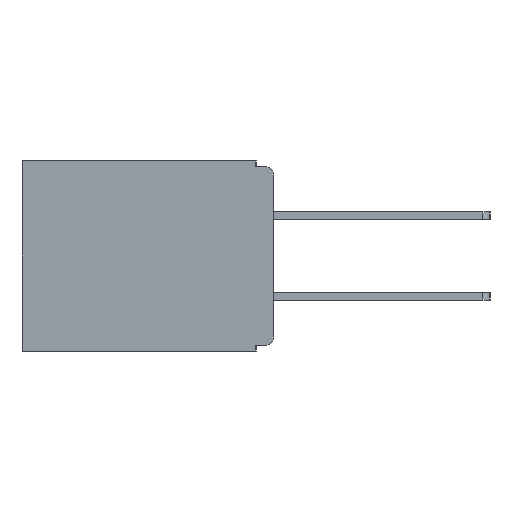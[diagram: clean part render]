
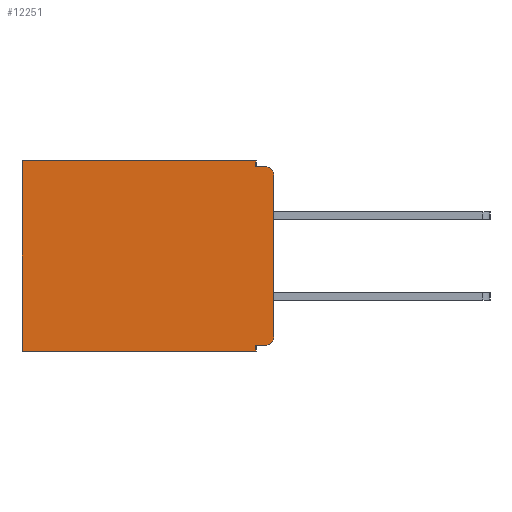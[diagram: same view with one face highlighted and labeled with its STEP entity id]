
A CAD part, left-side view. The second image highlights one B-rep face of the part: STEP entity #12251.
In plain terms, the highlighted planar face has unit normal (-1, 0, 0).
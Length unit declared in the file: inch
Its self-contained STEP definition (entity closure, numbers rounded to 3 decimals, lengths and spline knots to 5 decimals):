
#84 = AXIS2_PLACEMENT_3D ( 'NONE', #14376, #28313, #7454 ) ;
#860 = CARTESIAN_POINT ( 'NONE',  ( 0.3, 0.437, 0. ) ) ;
#1020 = DIRECTION ( 'NONE',  ( 0., 1., 0. ) ) ;
#1038 = CARTESIAN_POINT ( 'NONE',  ( 0.3, 0.015, -0.01 ) ) ;
#1476 = DIRECTION ( 'NONE',  ( 0., 0., -1. ) ) ;
#2027 = CARTESIAN_POINT ( 'NONE',  ( 0.3, 0.031, -0.32 ) ) ;
#2091 = EDGE_CURVE ( 'NONE', #27641, #7445, #16041, .T. ) ;
#2243 = CARTESIAN_POINT ( 'NONE',  ( 0.3, 0.031, -0.01 ) ) ;
#3721 = ORIENTED_EDGE ( 'NONE', *, *, #20288, .T. ) ;
#3724 = CARTESIAN_POINT ( 'NONE',  ( 0.3, 0., -0.33 ) ) ;
#3906 = VECTOR ( 'NONE', #7079, 39.37008 ) ;
#4555 = EDGE_CURVE ( 'NONE', #22523, #29433, #5527, .T. ) ;
#5527 = LINE ( 'NONE', #8312, #29497 ) ;
#5668 = CARTESIAN_POINT ( 'NONE',  ( 0.3, 0.437, -0.33 ) ) ;
#6530 = EDGE_CURVE ( 'NONE', #17334, #25809, #17372, .T. ) ;
#6709 = CARTESIAN_POINT ( 'NONE',  ( 0.3, 0.031, -0.33 ) ) ;
#6966 = DIRECTION ( 'NONE',  ( 0., 0., -1. ) ) ;
#7079 = DIRECTION ( 'NONE',  ( 0., -1., 0. ) ) ;
#7445 = VERTEX_POINT ( 'NONE', #1038 ) ;
#7454 = DIRECTION ( 'NONE',  ( 0., 0., -1. ) ) ;
#7565 = VERTEX_POINT ( 'NONE', #8309 ) ;
#8082 = VECTOR ( 'NONE', #24422, 39.37008 ) ;
#8164 = CARTESIAN_POINT ( 'NONE',  ( 0.3, 0., -0.33 ) ) ;
#8216 = AXIS2_PLACEMENT_3D ( 'NONE', #10210, #26488, #12535 ) ;
#8309 = CARTESIAN_POINT ( 'NONE',  ( 0.3, 0., -0.305 ) ) ;
#8312 = CARTESIAN_POINT ( 'NONE',  ( 0.3, 0., -0.32 ) ) ;
#9154 = LINE ( 'NONE', #12554, #20059 ) ;
#10089 = EDGE_CURVE ( 'NONE', #17334, #22535, #9154, .T. ) ;
#10210 = CARTESIAN_POINT ( 'NONE',  ( 0.3, 0.015, -0.305 ) ) ;
#10395 = ORIENTED_EDGE ( 'NONE', *, *, #4555, .F. ) ;
#10465 = FACE_OUTER_BOUND ( 'NONE', #14849, .T. ) ;
#11154 = VECTOR ( 'NONE', #16200, 39.37008 ) ;
#11649 = CARTESIAN_POINT ( 'NONE',  ( 0.3, 0., -0.01 ) ) ;
#12052 = ORIENTED_EDGE ( 'NONE', *, *, #26541, .T. ) ;
#12251 = ADVANCED_FACE ( 'NONE', ( #10465 ), #18564, .F. ) ;
#12495 = CARTESIAN_POINT ( 'NONE',  ( 0.3, 0.015, -0.32 ) ) ;
#12535 = DIRECTION ( 'NONE',  ( 0., 0., -1. ) ) ;
#12554 = CARTESIAN_POINT ( 'NONE',  ( 0.3, 0., 0. ) ) ;
#13854 = ORIENTED_EDGE ( 'NONE', *, *, #2091, .T. ) ;
#13874 = CARTESIAN_POINT ( 'NONE',  ( 0.3, 0., -0.33 ) ) ;
#14092 = VECTOR ( 'NONE', #1476, 39.37008 ) ;
#14376 = CARTESIAN_POINT ( 'NONE',  ( 0.3, 0.015, -0.025 ) ) ;
#14849 = EDGE_LOOP ( 'NONE', ( #21556, #13854, #17438, #26794, #24321, #3721, #17341, #28107, #10395, #12052 ) ) ;
#15052 = CARTESIAN_POINT ( 'NONE',  ( 0.3, 0.031, -0.33 ) ) ;
#15378 = EDGE_CURVE ( 'NONE', #23642, #28469, #19694, .T. ) ;
#15829 = CIRCLE ( 'NONE', #8216, 0.015 ) ;
#15917 = LINE ( 'NONE', #22423, #27546 ) ;
#16041 = CIRCLE ( 'NONE', #84, 0.015 ) ;
#16200 = DIRECTION ( 'NONE',  ( 0., 0., -1. ) ) ;
#16471 = CARTESIAN_POINT ( 'NONE',  ( 0.3, 0., -0.025 ) ) ;
#17334 = VERTEX_POINT ( 'NONE', #27373 ) ;
#17341 = ORIENTED_EDGE ( 'NONE', *, *, #15378, .F. ) ;
#17372 = LINE ( 'NONE', #27782, #11154 ) ;
#17438 = ORIENTED_EDGE ( 'NONE', *, *, #25849, .F. ) ;
#18564 = PLANE ( 'NONE',  #22810 ) ;
#19694 = LINE ( 'NONE', #8164, #8082 ) ;
#20059 = VECTOR ( 'NONE', #1020, 39.37008 ) ;
#20288 = EDGE_CURVE ( 'NONE', #22535, #28469, #15917, .T. ) ;
#20693 = LINE ( 'NONE', #6709, #25427 ) ;
#20875 = DIRECTION ( 'NONE',  ( 1., 0., 0. ) ) ;
#20979 = LINE ( 'NONE', #3724, #14092 ) ;
#21556 = ORIENTED_EDGE ( 'NONE', *, *, #25055, .F. ) ;
#22378 = LINE ( 'NONE', #11649, #3906 ) ;
#22423 = CARTESIAN_POINT ( 'NONE',  ( 0.3, 0.437, -0.33 ) ) ;
#22523 = VERTEX_POINT ( 'NONE', #12495 ) ;
#22535 = VERTEX_POINT ( 'NONE', #860 ) ;
#22810 = AXIS2_PLACEMENT_3D ( 'NONE', #13874, #20875, #6966 ) ;
#23291 = EDGE_CURVE ( 'NONE', #29433, #23642, #20693, .T. ) ;
#23642 = VERTEX_POINT ( 'NONE', #15052 ) ;
#24321 = ORIENTED_EDGE ( 'NONE', *, *, #10089, .T. ) ;
#24422 = DIRECTION ( 'NONE',  ( 0., 1., 0. ) ) ;
#24781 = DIRECTION ( 'NONE',  ( 0., 0., -1. ) ) ;
#25055 = EDGE_CURVE ( 'NONE', #27641, #7565, #20979, .T. ) ;
#25296 = DIRECTION ( 'NONE',  ( 0., 0., -1. ) ) ;
#25427 = VECTOR ( 'NONE', #25296, 39.37008 ) ;
#25809 = VERTEX_POINT ( 'NONE', #2243 ) ;
#25849 = EDGE_CURVE ( 'NONE', #25809, #7445, #22378, .T. ) ;
#26488 = DIRECTION ( 'NONE',  ( -1., 0., 0. ) ) ;
#26541 = EDGE_CURVE ( 'NONE', #22523, #7565, #15829, .T. ) ;
#26794 = ORIENTED_EDGE ( 'NONE', *, *, #6530, .F. ) ;
#27373 = CARTESIAN_POINT ( 'NONE',  ( 0.3, 0.031, 0. ) ) ;
#27546 = VECTOR ( 'NONE', #24781, 39.37008 ) ;
#27641 = VERTEX_POINT ( 'NONE', #16471 ) ;
#27782 = CARTESIAN_POINT ( 'NONE',  ( 0.3, 0.031, 0. ) ) ;
#27847 = DIRECTION ( 'NONE',  ( 0., 1., 0. ) ) ;
#28107 = ORIENTED_EDGE ( 'NONE', *, *, #23291, .F. ) ;
#28313 = DIRECTION ( 'NONE',  ( -1., 0., 0. ) ) ;
#28469 = VERTEX_POINT ( 'NONE', #5668 ) ;
#29433 = VERTEX_POINT ( 'NONE', #2027 ) ;
#29497 = VECTOR ( 'NONE', #27847, 39.37008 ) ;
